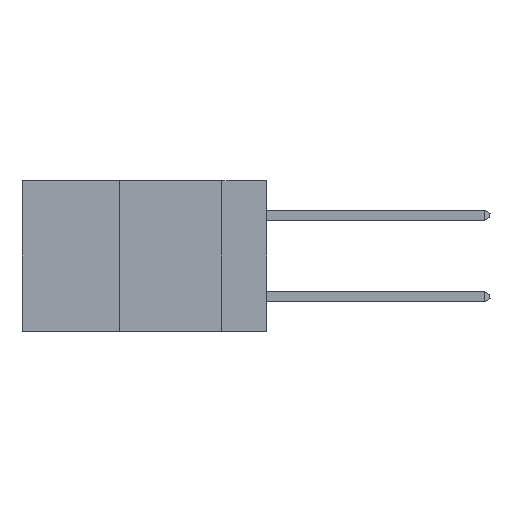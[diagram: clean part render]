
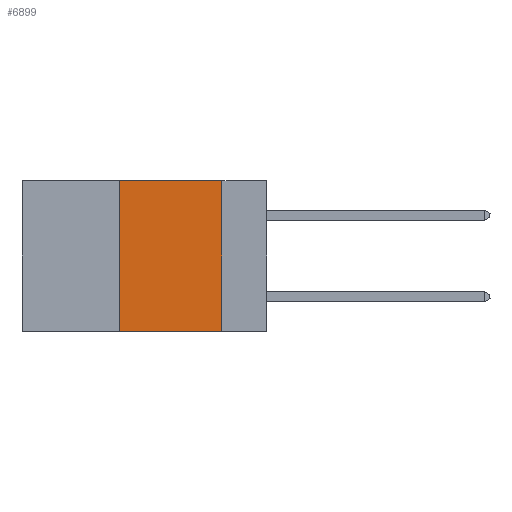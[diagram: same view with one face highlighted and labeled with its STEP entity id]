
A CAD part, left-side view. The second image highlights one B-rep face of the part: STEP entity #6899.
In plain terms, the highlighted planar face has unit normal (-1, 0, 0).
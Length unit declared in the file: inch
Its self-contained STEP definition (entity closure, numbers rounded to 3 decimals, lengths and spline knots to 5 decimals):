
#315 = CARTESIAN_POINT ( 'NONE',  ( 0., 0.6, 0. ) ) ;
#1201 = DIRECTION ( 'NONE',  ( 1., 0., 0. ) ) ;
#1257 = LINE ( 'NONE', #5613, #3341 ) ;
#1307 = CARTESIAN_POINT ( 'NONE',  ( 0., 0.11, 0. ) ) ;
#1365 = VERTEX_POINT ( 'NONE', #5181 ) ;
#2141 = ORIENTED_EDGE ( 'NONE', *, *, #8358, .F. ) ;
#2164 = DIRECTION ( 'NONE',  ( 0., -1., 0. ) ) ;
#2226 = DIRECTION ( 'NONE',  ( 0., 0., -1. ) ) ;
#2359 = VECTOR ( 'NONE', #2226, 39.37008 ) ;
#2406 = ORIENTED_EDGE ( 'NONE', *, *, #7640, .T. ) ;
#2449 = CARTESIAN_POINT ( 'NONE',  ( 0., 0.11, -0.37 ) ) ;
#2964 = EDGE_CURVE ( 'NONE', #8778, #3954, #4892, .T. ) ;
#3251 = DIRECTION ( 'NONE',  ( 0., -1., 0. ) ) ;
#3341 = VECTOR ( 'NONE', #2164, 39.37008 ) ;
#3584 = CARTESIAN_POINT ( 'NONE',  ( 0., 0.36, 0. ) ) ;
#3713 = CARTESIAN_POINT ( 'NONE',  ( 0., 0.36, 0. ) ) ;
#3954 = VERTEX_POINT ( 'NONE', #10598 ) ;
#4413 = CARTESIAN_POINT ( 'NONE',  ( 0., 0.6, 0. ) ) ;
#4892 = LINE ( 'NONE', #4413, #7251 ) ;
#5152 = VECTOR ( 'NONE', #8775, 39.37008 ) ;
#5181 = CARTESIAN_POINT ( 'NONE',  ( 0., 0.36, -0.37 ) ) ;
#5613 = CARTESIAN_POINT ( 'NONE',  ( 0., 0.6, -0.37 ) ) ;
#6475 = PLANE ( 'NONE',  #9497 ) ;
#6792 = ORIENTED_EDGE ( 'NONE', *, *, #2964, .F. ) ;
#6899 = ADVANCED_FACE ( 'NONE', ( #10572 ), #6475, .F. ) ;
#7094 = VERTEX_POINT ( 'NONE', #2449 ) ;
#7251 = VECTOR ( 'NONE', #3251, 39.37008 ) ;
#7331 = DIRECTION ( 'NONE',  ( 0., 0., -1. ) ) ;
#7492 = LINE ( 'NONE', #3713, #5152 ) ;
#7640 = EDGE_CURVE ( 'NONE', #1365, #7094, #1257, .T. ) ;
#8358 = EDGE_CURVE ( 'NONE', #3954, #7094, #9116, .T. ) ;
#8775 = DIRECTION ( 'NONE',  ( 0., 0., 1. ) ) ;
#8778 = VERTEX_POINT ( 'NONE', #3584 ) ;
#8921 = ORIENTED_EDGE ( 'NONE', *, *, #10073, .F. ) ;
#9116 = LINE ( 'NONE', #1307, #2359 ) ;
#9497 = AXIS2_PLACEMENT_3D ( 'NONE', #315, #1201, #7331 ) ;
#10073 = EDGE_CURVE ( 'NONE', #1365, #8778, #7492, .T. ) ;
#10140 = EDGE_LOOP ( 'NONE', ( #2141, #6792, #8921, #2406 ) ) ;
#10572 = FACE_OUTER_BOUND ( 'NONE', #10140, .T. ) ;
#10598 = CARTESIAN_POINT ( 'NONE',  ( 0., 0.11, 0. ) ) ;
